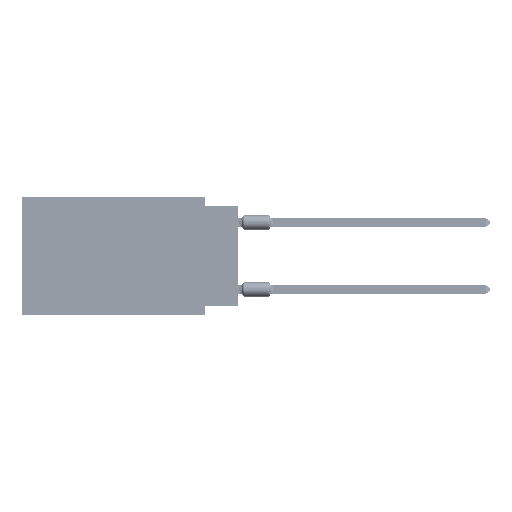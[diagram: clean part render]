
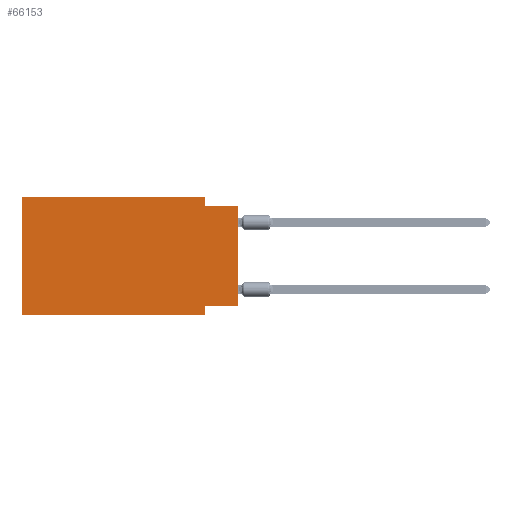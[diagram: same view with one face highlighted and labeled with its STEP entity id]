
A CAD part, left-side view. The second image highlights one B-rep face of the part: STEP entity #66153.
In plain terms, the highlighted planar face has unit normal (-1, 0, 0).
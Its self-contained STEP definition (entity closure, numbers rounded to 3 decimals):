
#1522 = LINE ( 'NONE', #84733, #35808 ) ;
#3688 = VECTOR ( 'NONE', #66727, 1000. ) ;
#4388 = VERTEX_POINT ( 'NONE', #12891 ) ;
#4872 = CARTESIAN_POINT ( 'NONE',  ( 0., 0., -8.255 ) ) ;
#9537 = ORIENTED_EDGE ( 'NONE', *, *, #53528, .T. ) ;
#10571 = ORIENTED_EDGE ( 'NONE', *, *, #16807, .T. ) ;
#10921 = ORIENTED_EDGE ( 'NONE', *, *, #60730, .F. ) ;
#12358 = VERTEX_POINT ( 'NONE', #47889 ) ;
#12891 = CARTESIAN_POINT ( 'NONE',  ( 0., 2.54, -8.255 ) ) ;
#13984 = DIRECTION ( 'NONE',  ( 0., 0., 1. ) ) ;
#15886 = VERTEX_POINT ( 'NONE', #86127 ) ;
#15966 = VERTEX_POINT ( 'NONE', #18355 ) ;
#16525 = VECTOR ( 'NONE', #24215, 1000. ) ;
#16807 = EDGE_CURVE ( 'NONE', #15966, #12358, #36402, .T. ) ;
#17294 = VERTEX_POINT ( 'NONE', #78404 ) ;
#18140 = LINE ( 'NONE', #89598, #3688 ) ;
#18355 = CARTESIAN_POINT ( 'NONE',  ( 0., 0., -8.255 ) ) ;
#18377 = ORIENTED_EDGE ( 'NONE', *, *, #28929, .F. ) ;
#18571 = PLANE ( 'NONE',  #78260 ) ;
#19841 = LINE ( 'NONE', #85994, #31544 ) ;
#20759 = DIRECTION ( 'NONE',  ( 0., 0., -1. ) ) ;
#21059 = VECTOR ( 'NONE', #86670, 1000. ) ;
#21589 = DIRECTION ( 'NONE',  ( 0., -1., 0. ) ) ;
#24215 = DIRECTION ( 'NONE',  ( 0., 0., 1. ) ) ;
#28929 = EDGE_CURVE ( 'NONE', #50579, #90059, #82565, .T. ) ;
#29474 = EDGE_CURVE ( 'NONE', #15886, #12358, #19841, .T. ) ;
#31544 = VECTOR ( 'NONE', #79909, 1000. ) ;
#33867 = LINE ( 'NONE', #4872, #52657 ) ;
#35139 = EDGE_LOOP ( 'NONE', ( #10571, #38834, #10921, #36203, #18377, #9537, #67275, #87939 ) ) ;
#35808 = VECTOR ( 'NONE', #20759, 1000. ) ;
#36203 = ORIENTED_EDGE ( 'NONE', *, *, #89240, .F. ) ;
#36402 = LINE ( 'NONE', #79818, #80935 ) ;
#38834 = ORIENTED_EDGE ( 'NONE', *, *, #29474, .F. ) ;
#41767 = DIRECTION ( 'NONE',  ( 0., 1., 0. ) ) ;
#44870 = VECTOR ( 'NONE', #21589, 1000. ) ;
#47057 = CARTESIAN_POINT ( 'NONE',  ( 0., 16.383, 0. ) ) ;
#47889 = CARTESIAN_POINT ( 'NONE',  ( 0., 0., -0.635 ) ) ;
#50292 = VERTEX_POINT ( 'NONE', #72084 ) ;
#50345 = EDGE_CURVE ( 'NONE', #4388, #50292, #1522, .T. ) ;
#50579 = VERTEX_POINT ( 'NONE', #75311 ) ;
#52657 = VECTOR ( 'NONE', #41767, 1000. ) ;
#53528 = EDGE_CURVE ( 'NONE', #50579, #50292, #57727, .T. ) ;
#56811 = CARTESIAN_POINT ( 'NONE',  ( 0., 16.383, -8.89 ) ) ;
#57727 = LINE ( 'NONE', #56811, #21059 ) ;
#60730 = EDGE_CURVE ( 'NONE', #17294, #15886, #18140, .T. ) ;
#63185 = EDGE_CURVE ( 'NONE', #15966, #4388, #33867, .T. ) ;
#66153 = ADVANCED_FACE ( 'NONE', ( #82552 ), #18571, .F. ) ;
#66727 = DIRECTION ( 'NONE',  ( 0., 0., -1. ) ) ;
#67275 = ORIENTED_EDGE ( 'NONE', *, *, #50345, .F. ) ;
#71338 = CARTESIAN_POINT ( 'NONE',  ( 0., 16.383, 0. ) ) ;
#72084 = CARTESIAN_POINT ( 'NONE',  ( 0., 2.54, -8.89 ) ) ;
#72481 = LINE ( 'NONE', #80399, #44870 ) ;
#75311 = CARTESIAN_POINT ( 'NONE',  ( 0., 16.383, -8.89 ) ) ;
#75546 = DIRECTION ( 'NONE',  ( 1., 0., 0. ) ) ;
#76920 = DIRECTION ( 'NONE',  ( 0., 0., -1. ) ) ;
#78260 = AXIS2_PLACEMENT_3D ( 'NONE', #47057, #75546, #76920 ) ;
#78404 = CARTESIAN_POINT ( 'NONE',  ( 0., 2.54, 0. ) ) ;
#79818 = CARTESIAN_POINT ( 'NONE',  ( 0., 0., 0. ) ) ;
#79909 = DIRECTION ( 'NONE',  ( 0., -1., 0. ) ) ;
#80399 = CARTESIAN_POINT ( 'NONE',  ( 0., 16.383, 0. ) ) ;
#80935 = VECTOR ( 'NONE', #13984, 1000. ) ;
#82552 = FACE_OUTER_BOUND ( 'NONE', #35139, .T. ) ;
#82565 = LINE ( 'NONE', #88673, #16525 ) ;
#84733 = CARTESIAN_POINT ( 'NONE',  ( 0., 2.54, -8.89 ) ) ;
#85994 = CARTESIAN_POINT ( 'NONE',  ( 0., 0., -0.635 ) ) ;
#86127 = CARTESIAN_POINT ( 'NONE',  ( 0., 2.54, -0.635 ) ) ;
#86670 = DIRECTION ( 'NONE',  ( 0., -1., 0. ) ) ;
#87939 = ORIENTED_EDGE ( 'NONE', *, *, #63185, .F. ) ;
#88673 = CARTESIAN_POINT ( 'NONE',  ( 0., 16.383, 0. ) ) ;
#89240 = EDGE_CURVE ( 'NONE', #90059, #17294, #72481, .T. ) ;
#89598 = CARTESIAN_POINT ( 'NONE',  ( 0., 2.54, 0. ) ) ;
#90059 = VERTEX_POINT ( 'NONE', #71338 ) ;
